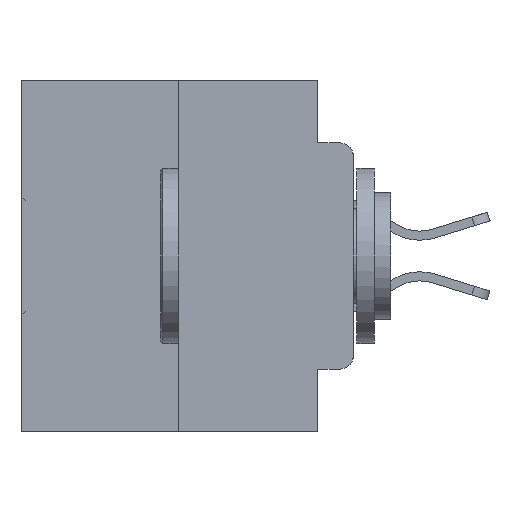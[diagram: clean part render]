
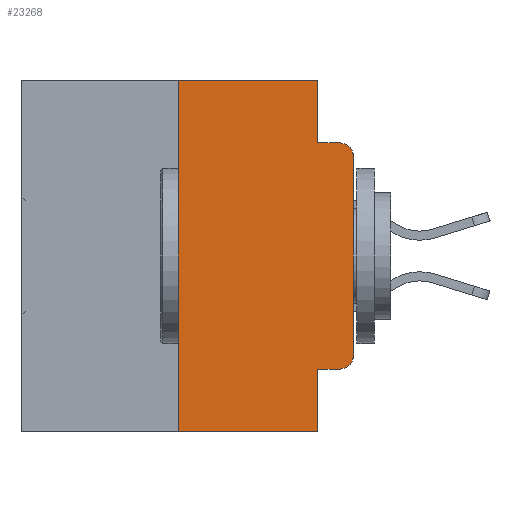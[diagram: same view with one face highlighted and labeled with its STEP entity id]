
A CAD part, left-side view. The second image highlights one B-rep face of the part: STEP entity #23268.
In plain terms, the highlighted planar face has unit normal (-1, 0, 0).
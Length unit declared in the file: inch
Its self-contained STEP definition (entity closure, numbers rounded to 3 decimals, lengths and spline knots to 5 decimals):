
#412 = EDGE_CURVE ( 'NONE', #6297, #13896, #29866, .T. ) ;
#881 = CIRCLE ( 'NONE', #26391, 0.02 ) ;
#1125 = DIRECTION ( 'NONE',  ( 0., -1., 0. ) ) ;
#1138 = CARTESIAN_POINT ( 'NONE',  ( 0., 0.02, -0.1085 ) ) ;
#1574 = CARTESIAN_POINT ( 'NONE',  ( 0., 0.051, -0.0885 ) ) ;
#2057 = FACE_OUTER_BOUND ( 'NONE', #31491, .T. ) ;
#2604 = CARTESIAN_POINT ( 'NONE',  ( 0., 0.051, 0. ) ) ;
#2639 = ORIENTED_EDGE ( 'NONE', *, *, #19983, .F. ) ;
#2949 = VERTEX_POINT ( 'NONE', #29325 ) ;
#3277 = VECTOR ( 'NONE', #23799, 39.37008 ) ;
#3735 = CARTESIAN_POINT ( 'NONE',  ( 0., 0.473, -0.5 ) ) ;
#3744 = DIRECTION ( 'NONE',  ( 0., 0., -1. ) ) ;
#4229 = CARTESIAN_POINT ( 'NONE',  ( 0., 0.25, 0. ) ) ;
#4254 = ORIENTED_EDGE ( 'NONE', *, *, #15092, .F. ) ;
#4552 = VECTOR ( 'NONE', #5219, 39.37008 ) ;
#4559 = CARTESIAN_POINT ( 'NONE',  ( 0., 0., 0. ) ) ;
#5219 = DIRECTION ( 'NONE',  ( 0., 0., -1. ) ) ;
#5833 = CARTESIAN_POINT ( 'NONE',  ( 0., 0.25, -0.5 ) ) ;
#6118 = EDGE_CURVE ( 'NONE', #13896, #6729, #881, .T. ) ;
#6297 = VERTEX_POINT ( 'NONE', #31709 ) ;
#6567 = DIRECTION ( 'NONE',  ( 0., 0., -1. ) ) ;
#6690 = EDGE_CURVE ( 'NONE', #20529, #28586, #30557, .T. ) ;
#6729 = VERTEX_POINT ( 'NONE', #16188 ) ;
#6866 = DIRECTION ( 'NONE',  ( 0., 0., 1. ) ) ;
#7233 = AXIS2_PLACEMENT_3D ( 'NONE', #1138, #18535, #3744 ) ;
#7382 = EDGE_CURVE ( 'NONE', #29280, #10127, #31617, .T. ) ;
#8716 = DIRECTION ( 'NONE',  ( 1., 0., 0. ) ) ;
#9738 = LINE ( 'NONE', #27041, #15438 ) ;
#9961 = LINE ( 'NONE', #1574, #3277 ) ;
#10127 = VERTEX_POINT ( 'NONE', #4229 ) ;
#11286 = ORIENTED_EDGE ( 'NONE', *, *, #6118, .T. ) ;
#11635 = DIRECTION ( 'NONE',  ( -1., 0., 0. ) ) ;
#12475 = DIRECTION ( 'NONE',  ( 0., -1., 0. ) ) ;
#13540 = ORIENTED_EDGE ( 'NONE', *, *, #6690, .T. ) ;
#13827 = CARTESIAN_POINT ( 'NONE',  ( 0., 0.051, 0. ) ) ;
#13888 = EDGE_CURVE ( 'NONE', #6729, #20529, #24986, .T. ) ;
#13896 = VERTEX_POINT ( 'NONE', #29092 ) ;
#13956 = ORIENTED_EDGE ( 'NONE', *, *, #27116, .T. ) ;
#14688 = ORIENTED_EDGE ( 'NONE', *, *, #29821, .F. ) ;
#15092 = EDGE_CURVE ( 'NONE', #10127, #18406, #9738, .T. ) ;
#15438 = VECTOR ( 'NONE', #12475, 39.37008 ) ;
#16188 = CARTESIAN_POINT ( 'NONE',  ( 0., 0., -0.3915 ) ) ;
#16247 = ORIENTED_EDGE ( 'NONE', *, *, #412, .T. ) ;
#16381 = CARTESIAN_POINT ( 'NONE',  ( 0., 0.051, -0.4115 ) ) ;
#17471 = CARTESIAN_POINT ( 'NONE',  ( 0., 0., -0.1085 ) ) ;
#17667 = LINE ( 'NONE', #2604, #4552 ) ;
#17769 = VECTOR ( 'NONE', #1125, 39.37008 ) ;
#18381 = PLANE ( 'NONE',  #21585 ) ;
#18406 = VERTEX_POINT ( 'NONE', #25302 ) ;
#18504 = VERTEX_POINT ( 'NONE', #27939 ) ;
#18535 = DIRECTION ( 'NONE',  ( -1., 0., 0. ) ) ;
#18910 = ORIENTED_EDGE ( 'NONE', *, *, #7382, .F. ) ;
#19279 = DIRECTION ( 'NONE',  ( 0., 0., 1. ) ) ;
#19983 = EDGE_CURVE ( 'NONE', #18504, #28586, #9961, .T. ) ;
#20023 = LINE ( 'NONE', #3735, #17769 ) ;
#20529 = VERTEX_POINT ( 'NONE', #17471 ) ;
#20789 = CARTESIAN_POINT ( 'NONE',  ( 0., 0.473, 0. ) ) ;
#21585 = AXIS2_PLACEMENT_3D ( 'NONE', #20789, #8716, #25719 ) ;
#22864 = LINE ( 'NONE', #13827, #27793 ) ;
#23268 = ADVANCED_FACE ( 'NONE', ( #2057 ), #18381, .F. ) ;
#23799 = DIRECTION ( 'NONE',  ( 0., -1., 0. ) ) ;
#24962 = ORIENTED_EDGE ( 'NONE', *, *, #13888, .T. ) ;
#24986 = LINE ( 'NONE', #4559, #31443 ) ;
#25302 = CARTESIAN_POINT ( 'NONE',  ( 0., 0.051, 0. ) ) ;
#25719 = DIRECTION ( 'NONE',  ( 0., 0., -1. ) ) ;
#26210 = CARTESIAN_POINT ( 'NONE',  ( 0., 0.02, -0.3915 ) ) ;
#26255 = CARTESIAN_POINT ( 'NONE',  ( 0., 0.25, 0. ) ) ;
#26391 = AXIS2_PLACEMENT_3D ( 'NONE', #26210, #11635, #28659 ) ;
#26686 = VECTOR ( 'NONE', #6866, 39.37008 ) ;
#27004 = DIRECTION ( 'NONE',  ( 0., -1., 0. ) ) ;
#27041 = CARTESIAN_POINT ( 'NONE',  ( 0., 0.473, 0. ) ) ;
#27116 = EDGE_CURVE ( 'NONE', #29280, #2949, #20023, .T. ) ;
#27793 = VECTOR ( 'NONE', #6567, 39.37008 ) ;
#27939 = CARTESIAN_POINT ( 'NONE',  ( 0., 0.051, -0.0885 ) ) ;
#28586 = VERTEX_POINT ( 'NONE', #31917 ) ;
#28659 = DIRECTION ( 'NONE',  ( 0., 0., -1. ) ) ;
#29084 = VECTOR ( 'NONE', #27004, 39.37008 ) ;
#29092 = CARTESIAN_POINT ( 'NONE',  ( 0., 0.02, -0.4115 ) ) ;
#29280 = VERTEX_POINT ( 'NONE', #5833 ) ;
#29325 = CARTESIAN_POINT ( 'NONE',  ( 0., 0.051, -0.5 ) ) ;
#29579 = ORIENTED_EDGE ( 'NONE', *, *, #31392, .F. ) ;
#29821 = EDGE_CURVE ( 'NONE', #6297, #2949, #17667, .T. ) ;
#29866 = LINE ( 'NONE', #16381, #29084 ) ;
#30557 = CIRCLE ( 'NONE', #7233, 0.02 ) ;
#31392 = EDGE_CURVE ( 'NONE', #18406, #18504, #22864, .T. ) ;
#31443 = VECTOR ( 'NONE', #19279, 39.37008 ) ;
#31491 = EDGE_LOOP ( 'NONE', ( #24962, #13540, #2639, #29579, #4254, #18910, #13956, #14688, #16247, #11286 ) ) ;
#31617 = LINE ( 'NONE', #26255, #26686 ) ;
#31709 = CARTESIAN_POINT ( 'NONE',  ( 0., 0.051, -0.4115 ) ) ;
#31917 = CARTESIAN_POINT ( 'NONE',  ( 0., 0.02, -0.0885 ) ) ;
